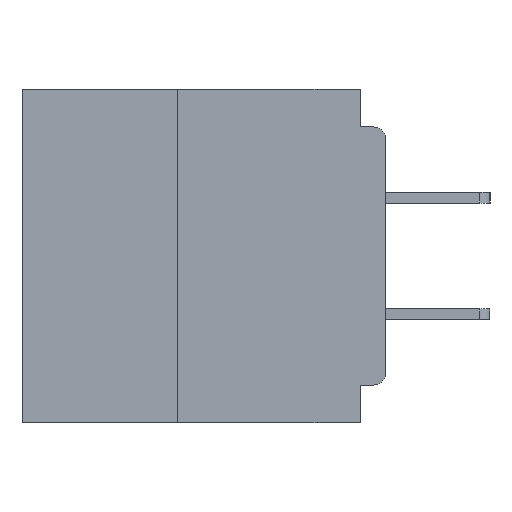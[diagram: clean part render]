
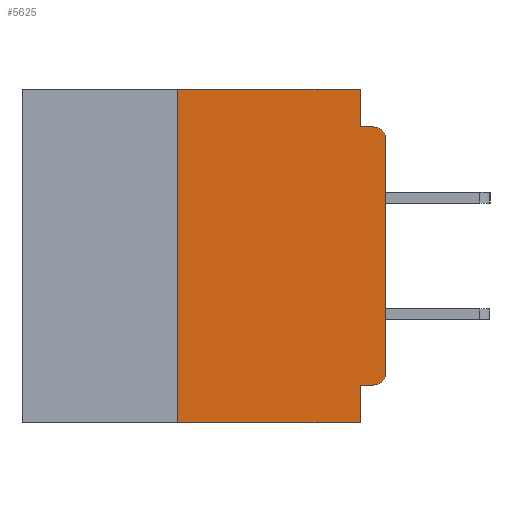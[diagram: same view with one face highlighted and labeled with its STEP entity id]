
A CAD part, left-side view. The second image highlights one B-rep face of the part: STEP entity #5625.
In plain terms, the highlighted planar face has unit normal (-1, 0, 0).
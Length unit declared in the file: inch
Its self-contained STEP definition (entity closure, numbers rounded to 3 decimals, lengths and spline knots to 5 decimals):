
#45 = DIRECTION ( 'NONE',  ( 0., 0., -1. ) ) ;
#541 = LINE ( 'NONE', #32682, #18076 ) ;
#657 = CIRCLE ( 'NONE', #30662, 0.015 ) ;
#1497 = EDGE_CURVE ( 'NONE', #11679, #24299, #19285, .T. ) ;
#1845 = VERTEX_POINT ( 'NONE', #13493 ) ;
#1957 = CARTESIAN_POINT ( 'NONE',  ( 0., 0.031, 0. ) ) ;
#2408 = EDGE_LOOP ( 'NONE', ( #39395, #18165, #20866, #39920, #17981, #30781, #11039, #14374, #10304, #6788 ) ) ;
#3377 = VERTEX_POINT ( 'NONE', #13230 ) ;
#4358 = EDGE_CURVE ( 'NONE', #24299, #11322, #40854, .T. ) ;
#5625 = ADVANCED_FACE ( 'NONE', ( #8393 ), #38174, .F. ) ;
#6788 = ORIENTED_EDGE ( 'NONE', *, *, #8912, .T. ) ;
#7923 = DIRECTION ( 'NONE',  ( 0., 0., -1. ) ) ;
#8309 = CARTESIAN_POINT ( 'NONE',  ( 0., 0., 0. ) ) ;
#8393 = FACE_OUTER_BOUND ( 'NONE', #2408, .T. ) ;
#8912 = EDGE_CURVE ( 'NONE', #3377, #11679, #657, .T. ) ;
#10133 = VECTOR ( 'NONE', #18050, 39.37008 ) ;
#10228 = VECTOR ( 'NONE', #19673, 39.37008 ) ;
#10304 = ORIENTED_EDGE ( 'NONE', *, *, #43991, .F. ) ;
#10684 = DIRECTION ( 'NONE',  ( 0., -1., 0. ) ) ;
#10866 = VECTOR ( 'NONE', #28542, 39.37008 ) ;
#11039 = ORIENTED_EDGE ( 'NONE', *, *, #22454, .T. ) ;
#11189 = LINE ( 'NONE', #35143, #10133 ) ;
#11279 = LINE ( 'NONE', #16171, #10228 ) ;
#11322 = VERTEX_POINT ( 'NONE', #41515 ) ;
#11423 = CARTESIAN_POINT ( 'NONE',  ( 0., 0.031, -0.045 ) ) ;
#11438 = EDGE_CURVE ( 'NONE', #19003, #42431, #31969, .T. ) ;
#11679 = VERTEX_POINT ( 'NONE', #33422 ) ;
#13230 = CARTESIAN_POINT ( 'NONE',  ( 0., 0.015, -0.355 ) ) ;
#13493 = CARTESIAN_POINT ( 'NONE',  ( 0., 0.25, 0. ) ) ;
#13665 = VECTOR ( 'NONE', #7923, 39.37008 ) ;
#13741 = AXIS2_PLACEMENT_3D ( 'NONE', #33618, #33427, #33379 ) ;
#14374 = ORIENTED_EDGE ( 'NONE', *, *, #11438, .F. ) ;
#14792 = CARTESIAN_POINT ( 'NONE',  ( 0., 0.031, -0.4 ) ) ;
#14840 = CARTESIAN_POINT ( 'NONE',  ( 0., 0., -0.045 ) ) ;
#16171 = CARTESIAN_POINT ( 'NONE',  ( 0., 0., -0.355 ) ) ;
#17154 = LINE ( 'NONE', #14840, #34357 ) ;
#17981 = ORIENTED_EDGE ( 'NONE', *, *, #31432, .F. ) ;
#18050 = DIRECTION ( 'NONE',  ( 0., 0., 1. ) ) ;
#18076 = VECTOR ( 'NONE', #39559, 39.37008 ) ;
#18165 = ORIENTED_EDGE ( 'NONE', *, *, #4358, .T. ) ;
#18433 = CARTESIAN_POINT ( 'NONE',  ( 0., 0.031, -0.4 ) ) ;
#18477 = DIRECTION ( 'NONE',  ( 0., 0., 1. ) ) ;
#18970 = VECTOR ( 'NONE', #10684, 39.37008 ) ;
#19003 = VERTEX_POINT ( 'NONE', #25609 ) ;
#19285 = LINE ( 'NONE', #8309, #39541 ) ;
#19673 = DIRECTION ( 'NONE',  ( 0., 1., 0. ) ) ;
#20751 = EDGE_CURVE ( 'NONE', #28695, #11322, #17154, .T. ) ;
#20866 = ORIENTED_EDGE ( 'NONE', *, *, #20751, .F. ) ;
#21014 = DIRECTION ( 'NONE',  ( -1., 0., 0. ) ) ;
#21644 = CARTESIAN_POINT ( 'NONE',  ( 0., 0., -0.06 ) ) ;
#21846 = DIRECTION ( 'NONE',  ( 0., -1., 0. ) ) ;
#22454 = EDGE_CURVE ( 'NONE', #40160, #42431, #541, .T. ) ;
#24299 = VERTEX_POINT ( 'NONE', #21644 ) ;
#25122 = CARTESIAN_POINT ( 'NONE',  ( 0., 0.031, 0. ) ) ;
#25609 = CARTESIAN_POINT ( 'NONE',  ( 0., 0.031, -0.355 ) ) ;
#28542 = DIRECTION ( 'NONE',  ( 0., 0., -1. ) ) ;
#28695 = VERTEX_POINT ( 'NONE', #11423 ) ;
#30662 = AXIS2_PLACEMENT_3D ( 'NONE', #41487, #21014, #45 ) ;
#30781 = ORIENTED_EDGE ( 'NONE', *, *, #39489, .F. ) ;
#31432 = EDGE_CURVE ( 'NONE', #1845, #34558, #37187, .T. ) ;
#31697 = AXIS2_PLACEMENT_3D ( 'NONE', #38973, #37908, #37007 ) ;
#31969 = LINE ( 'NONE', #14792, #13665 ) ;
#32682 = CARTESIAN_POINT ( 'NONE',  ( 0., 0.437, -0.4 ) ) ;
#33379 = DIRECTION ( 'NONE',  ( 0., 0., -1. ) ) ;
#33422 = CARTESIAN_POINT ( 'NONE',  ( 0., 0., -0.34 ) ) ;
#33427 = DIRECTION ( 'NONE',  ( -1., 0., 0. ) ) ;
#33618 = CARTESIAN_POINT ( 'NONE',  ( 0., 0.015, -0.06 ) ) ;
#34357 = VECTOR ( 'NONE', #21846, 39.37008 ) ;
#34558 = VERTEX_POINT ( 'NONE', #1957 ) ;
#34774 = CARTESIAN_POINT ( 'NONE',  ( 0., 0.437, 0. ) ) ;
#35143 = CARTESIAN_POINT ( 'NONE',  ( 0., 0.25, -0.4 ) ) ;
#35405 = CARTESIAN_POINT ( 'NONE',  ( 0., 0.25, -0.4 ) ) ;
#36548 = EDGE_CURVE ( 'NONE', #34558, #28695, #38345, .T. ) ;
#37007 = DIRECTION ( 'NONE',  ( 0., 0., -1. ) ) ;
#37187 = LINE ( 'NONE', #34774, #18970 ) ;
#37908 = DIRECTION ( 'NONE',  ( 1., 0., 0. ) ) ;
#38174 = PLANE ( 'NONE',  #31697 ) ;
#38345 = LINE ( 'NONE', #25122, #10866 ) ;
#38973 = CARTESIAN_POINT ( 'NONE',  ( 0., 0.437, 0. ) ) ;
#39395 = ORIENTED_EDGE ( 'NONE', *, *, #1497, .T. ) ;
#39489 = EDGE_CURVE ( 'NONE', #40160, #1845, #11189, .T. ) ;
#39541 = VECTOR ( 'NONE', #18477, 39.37008 ) ;
#39559 = DIRECTION ( 'NONE',  ( 0., -1., 0. ) ) ;
#39920 = ORIENTED_EDGE ( 'NONE', *, *, #36548, .F. ) ;
#40160 = VERTEX_POINT ( 'NONE', #35405 ) ;
#40854 = CIRCLE ( 'NONE', #13741, 0.015 ) ;
#41487 = CARTESIAN_POINT ( 'NONE',  ( 0., 0.015, -0.34 ) ) ;
#41515 = CARTESIAN_POINT ( 'NONE',  ( 0., 0.015, -0.045 ) ) ;
#42431 = VERTEX_POINT ( 'NONE', #18433 ) ;
#43991 = EDGE_CURVE ( 'NONE', #3377, #19003, #11279, .T. ) ;
